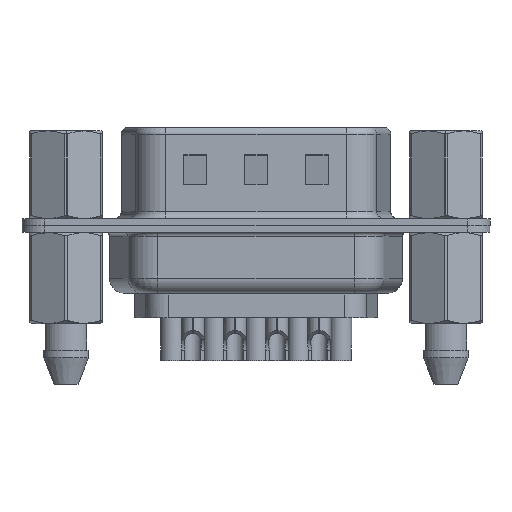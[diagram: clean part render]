
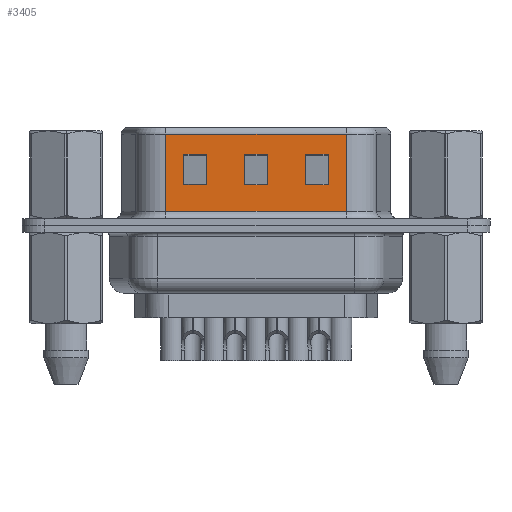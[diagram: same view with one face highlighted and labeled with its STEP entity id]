
A CAD part, front view. The second image highlights one B-rep face of the part: STEP entity #3405.
In plain terms, the highlighted planar face has unit normal (0, -1, 0).
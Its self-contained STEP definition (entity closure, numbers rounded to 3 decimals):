
#42 = DIRECTION ( 'NONE',  ( 0., 0., -1. ) ) ;
#59 = VERTEX_POINT ( 'NONE', #491 ) ;
#119 = EDGE_LOOP ( 'NONE', ( #10452, #9525, #20801, #19667 ) ) ;
#145 = VERTEX_POINT ( 'NONE', #14780 ) ;
#148 = VERTEX_POINT ( 'NONE', #18341 ) ;
#491 = CARTESIAN_POINT ( 'NONE',  ( 15.745, -4.58, 2.705 ) ) ;
#794 = PLANE ( 'NONE',  #2396 ) ;
#1153 = EDGE_CURVE ( 'NONE', #14087, #14114, #21390, .T. ) ;
#1272 = DIRECTION ( 'NONE',  ( 1., 0., 0. ) ) ;
#1362 = EDGE_LOOP ( 'NONE', ( #4995, #13405, #9549, #3657 ) ) ;
#1523 = VERTEX_POINT ( 'NONE', #17442 ) ;
#1812 = CARTESIAN_POINT ( 'NONE',  ( 11.745, -4.58, 2.705 ) ) ;
#2087 = EDGE_LOOP ( 'NONE', ( #8774, #13832, #21997, #5401 ) ) ;
#2187 = VERTEX_POINT ( 'NONE', #4568 ) ;
#2296 = CARTESIAN_POINT ( 'NONE',  ( 18.445, -4.58, 4.705 ) ) ;
#2396 = AXIS2_PLACEMENT_3D ( 'NONE', #7499, #9267, #7608 ) ;
#2771 = VECTOR ( 'NONE', #11602, 1000. ) ;
#2872 = CARTESIAN_POINT ( 'NONE',  ( 11.745, -4.58, 6.52 ) ) ;
#2961 = CARTESIAN_POINT ( 'NONE',  ( 17.245, -4.58, 6.52 ) ) ;
#3309 = LINE ( 'NONE', #2872, #2771 ) ;
#3405 = ADVANCED_FACE ( 'NONE', ( #17311, #13974, #17418, #4128 ), #794, .F. ) ;
#3531 = ORIENTED_EDGE ( 'NONE', *, *, #12046, .T. ) ;
#3657 = ORIENTED_EDGE ( 'NONE', *, *, #21316, .T. ) ;
#3838 = EDGE_CURVE ( 'NONE', #145, #2187, #11483, .T. ) ;
#4119 = VECTOR ( 'NONE', #16813, 1000. ) ;
#4128 = FACE_OUTER_BOUND ( 'NONE', #119, .T. ) ;
#4151 = VERTEX_POINT ( 'NONE', #11558 ) ;
#4568 = CARTESIAN_POINT ( 'NONE',  ( 17.245, -4.58, 2.705 ) ) ;
#4668 = EDGE_CURVE ( 'NONE', #2187, #59, #5708, .T. ) ;
#4843 = VECTOR ( 'NONE', #10583, 1000. ) ;
#4961 = CARTESIAN_POINT ( 'NONE',  ( 15.745, -4.58, 6.52 ) ) ;
#4995 = ORIENTED_EDGE ( 'NONE', *, *, #3838, .T. ) ;
#5028 = CARTESIAN_POINT ( 'NONE',  ( 7.745, -4.58, 2.705 ) ) ;
#5157 = LINE ( 'NONE', #18678, #11445 ) ;
#5159 = CARTESIAN_POINT ( 'NONE',  ( 6.545, -4.58, 0.95 ) ) ;
#5401 = ORIENTED_EDGE ( 'NONE', *, *, #1153, .T. ) ;
#5708 = LINE ( 'NONE', #19339, #16748 ) ;
#6379 = VECTOR ( 'NONE', #9456, 1000. ) ;
#6510 = DIRECTION ( 'NONE',  ( 1., 0., 0. ) ) ;
#7076 = VERTEX_POINT ( 'NONE', #19908 ) ;
#7185 = DIRECTION ( 'NONE',  ( 0., 0., -1. ) ) ;
#7499 = CARTESIAN_POINT ( 'NONE',  ( 18.445, -4.58, 6.52 ) ) ;
#7608 = DIRECTION ( 'NONE',  ( 0., 0., 1. ) ) ;
#7680 = DIRECTION ( 'NONE',  ( 1., 0., 0. ) ) ;
#7940 = VERTEX_POINT ( 'NONE', #14872 ) ;
#8027 = LINE ( 'NONE', #18307, #21041 ) ;
#8086 = VERTEX_POINT ( 'NONE', #5028 ) ;
#8141 = DIRECTION ( 'NONE',  ( -1., 0., 0. ) ) ;
#8223 = LINE ( 'NONE', #19634, #6379 ) ;
#8225 = VECTOR ( 'NONE', #13385, 1000. ) ;
#8244 = CARTESIAN_POINT ( 'NONE',  ( 13.245, -4.58, 6.52 ) ) ;
#8504 = VECTOR ( 'NONE', #6510, 1000. ) ;
#8774 = ORIENTED_EDGE ( 'NONE', *, *, #19474, .T. ) ;
#8834 = EDGE_LOOP ( 'NONE', ( #16763, #3531, #20374, #21384 ) ) ;
#9267 = DIRECTION ( 'NONE',  ( 0., 1., 0. ) ) ;
#9456 = DIRECTION ( 'NONE',  ( 0., 0., 1. ) ) ;
#9525 = ORIENTED_EDGE ( 'NONE', *, *, #10817, .T. ) ;
#9549 = ORIENTED_EDGE ( 'NONE', *, *, #17014, .T. ) ;
#9555 = VECTOR ( 'NONE', #11391, 1000. ) ;
#10452 = ORIENTED_EDGE ( 'NONE', *, *, #16997, .F. ) ;
#10583 = DIRECTION ( 'NONE',  ( -1., 0., 0. ) ) ;
#10817 = EDGE_CURVE ( 'NONE', #1523, #7076, #19079, .T. ) ;
#11391 = DIRECTION ( 'NONE',  ( 0., 0., -1. ) ) ;
#11411 = VECTOR ( 'NONE', #18409, 1000. ) ;
#11445 = VECTOR ( 'NONE', #7185, 1000. ) ;
#11483 = LINE ( 'NONE', #2961, #14759 ) ;
#11558 = CARTESIAN_POINT ( 'NONE',  ( 18.445, -4.58, 0.95 ) ) ;
#11602 = DIRECTION ( 'NONE',  ( 0., 0., 1. ) ) ;
#11612 = LINE ( 'NONE', #13075, #11411 ) ;
#11705 = EDGE_CURVE ( 'NONE', #7076, #12458, #5157, .T. ) ;
#11898 = LINE ( 'NONE', #15361, #13750 ) ;
#12046 = EDGE_CURVE ( 'NONE', #21597, #7940, #21888, .T. ) ;
#12079 = CARTESIAN_POINT ( 'NONE',  ( 7.745, -4.58, 4.705 ) ) ;
#12458 = VERTEX_POINT ( 'NONE', #5159 ) ;
#12874 = DIRECTION ( 'NONE',  ( -1., 0., 0. ) ) ;
#12910 = CARTESIAN_POINT ( 'NONE',  ( 14.445, -4.58, 4.705 ) ) ;
#13075 = CARTESIAN_POINT ( 'NONE',  ( 18.445, -4.58, 0.95 ) ) ;
#13229 = LINE ( 'NONE', #16569, #20305 ) ;
#13354 = LINE ( 'NONE', #4961, #4119 ) ;
#13385 = DIRECTION ( 'NONE',  ( 0., 0., -1. ) ) ;
#13405 = ORIENTED_EDGE ( 'NONE', *, *, #4668, .T. ) ;
#13663 = EDGE_CURVE ( 'NONE', #8086, #14087, #8223, .T. ) ;
#13750 = VECTOR ( 'NONE', #42, 1000. ) ;
#13832 = ORIENTED_EDGE ( 'NONE', *, *, #21198, .T. ) ;
#13974 = FACE_BOUND ( 'NONE', #1362, .T. ) ;
#14087 = VERTEX_POINT ( 'NONE', #12079 ) ;
#14114 = VERTEX_POINT ( 'NONE', #17216 ) ;
#14338 = EDGE_CURVE ( 'NONE', #7940, #18689, #8027, .T. ) ;
#14340 = EDGE_CURVE ( 'NONE', #12458, #4151, #11612, .T. ) ;
#14442 = EDGE_CURVE ( 'NONE', #148, #21597, #17719, .T. ) ;
#14466 = CARTESIAN_POINT ( 'NONE',  ( 9.245, -4.58, 2.705 ) ) ;
#14759 = VECTOR ( 'NONE', #18065, 1000. ) ;
#14780 = CARTESIAN_POINT ( 'NONE',  ( 17.245, -4.58, 4.705 ) ) ;
#14872 = CARTESIAN_POINT ( 'NONE',  ( 13.245, -4.58, 2.705 ) ) ;
#15361 = CARTESIAN_POINT ( 'NONE',  ( 18.445, -4.58, 6.52 ) ) ;
#16122 = VERTEX_POINT ( 'NONE', #18074 ) ;
#16152 = DIRECTION ( 'NONE',  ( -1., 0., 0. ) ) ;
#16202 = CARTESIAN_POINT ( 'NONE',  ( 13.245, -4.58, 4.705 ) ) ;
#16412 = CARTESIAN_POINT ( 'NONE',  ( 9.245, -4.58, 6.52 ) ) ;
#16569 = CARTESIAN_POINT ( 'NONE',  ( 22.445, -4.58, 4.705 ) ) ;
#16748 = VECTOR ( 'NONE', #12874, 1000. ) ;
#16763 = ORIENTED_EDGE ( 'NONE', *, *, #14442, .T. ) ;
#16813 = DIRECTION ( 'NONE',  ( 0., 0., 1. ) ) ;
#16997 = EDGE_CURVE ( 'NONE', #1523, #4151, #11898, .T. ) ;
#17014 = EDGE_CURVE ( 'NONE', #59, #16122, #13354, .T. ) ;
#17216 = CARTESIAN_POINT ( 'NONE',  ( 9.245, -4.58, 4.705 ) ) ;
#17311 = FACE_BOUND ( 'NONE', #2087, .T. ) ;
#17418 = FACE_BOUND ( 'NONE', #8834, .T. ) ;
#17442 = CARTESIAN_POINT ( 'NONE',  ( 18.445, -4.58, 6.02 ) ) ;
#17719 = LINE ( 'NONE', #2296, #19630 ) ;
#18065 = DIRECTION ( 'NONE',  ( 0., 0., -1. ) ) ;
#18074 = CARTESIAN_POINT ( 'NONE',  ( 15.745, -4.58, 4.705 ) ) ;
#18307 = CARTESIAN_POINT ( 'NONE',  ( 18.445, -4.58, 2.705 ) ) ;
#18341 = CARTESIAN_POINT ( 'NONE',  ( 11.745, -4.58, 4.705 ) ) ;
#18409 = DIRECTION ( 'NONE',  ( 1., 0., 0. ) ) ;
#18509 = LINE ( 'NONE', #16412, #9555 ) ;
#18678 = CARTESIAN_POINT ( 'NONE',  ( 6.545, -4.58, 6.52 ) ) ;
#18689 = VERTEX_POINT ( 'NONE', #1812 ) ;
#19079 = LINE ( 'NONE', #19311, #4843 ) ;
#19311 = CARTESIAN_POINT ( 'NONE',  ( 18.445, -4.58, 6.02 ) ) ;
#19339 = CARTESIAN_POINT ( 'NONE',  ( 22.445, -4.58, 2.705 ) ) ;
#19474 = EDGE_CURVE ( 'NONE', #14114, #21250, #18509, .T. ) ;
#19501 = EDGE_CURVE ( 'NONE', #18689, #148, #3309, .T. ) ;
#19597 = VECTOR ( 'NONE', #16152, 1000. ) ;
#19599 = LINE ( 'NONE', #19808, #19597 ) ;
#19630 = VECTOR ( 'NONE', #7680, 1000. ) ;
#19634 = CARTESIAN_POINT ( 'NONE',  ( 7.745, -4.58, 6.52 ) ) ;
#19667 = ORIENTED_EDGE ( 'NONE', *, *, #14340, .T. ) ;
#19808 = CARTESIAN_POINT ( 'NONE',  ( 14.445, -4.58, 2.705 ) ) ;
#19908 = CARTESIAN_POINT ( 'NONE',  ( 6.545, -4.58, 6.02 ) ) ;
#20305 = VECTOR ( 'NONE', #1272, 1000. ) ;
#20374 = ORIENTED_EDGE ( 'NONE', *, *, #14338, .T. ) ;
#20801 = ORIENTED_EDGE ( 'NONE', *, *, #11705, .T. ) ;
#21041 = VECTOR ( 'NONE', #8141, 1000. ) ;
#21198 = EDGE_CURVE ( 'NONE', #21250, #8086, #19599, .T. ) ;
#21250 = VERTEX_POINT ( 'NONE', #14466 ) ;
#21316 = EDGE_CURVE ( 'NONE', #16122, #145, #13229, .T. ) ;
#21384 = ORIENTED_EDGE ( 'NONE', *, *, #19501, .T. ) ;
#21390 = LINE ( 'NONE', #12910, #8504 ) ;
#21597 = VERTEX_POINT ( 'NONE', #16202 ) ;
#21888 = LINE ( 'NONE', #8244, #8225 ) ;
#21997 = ORIENTED_EDGE ( 'NONE', *, *, #13663, .T. ) ;
